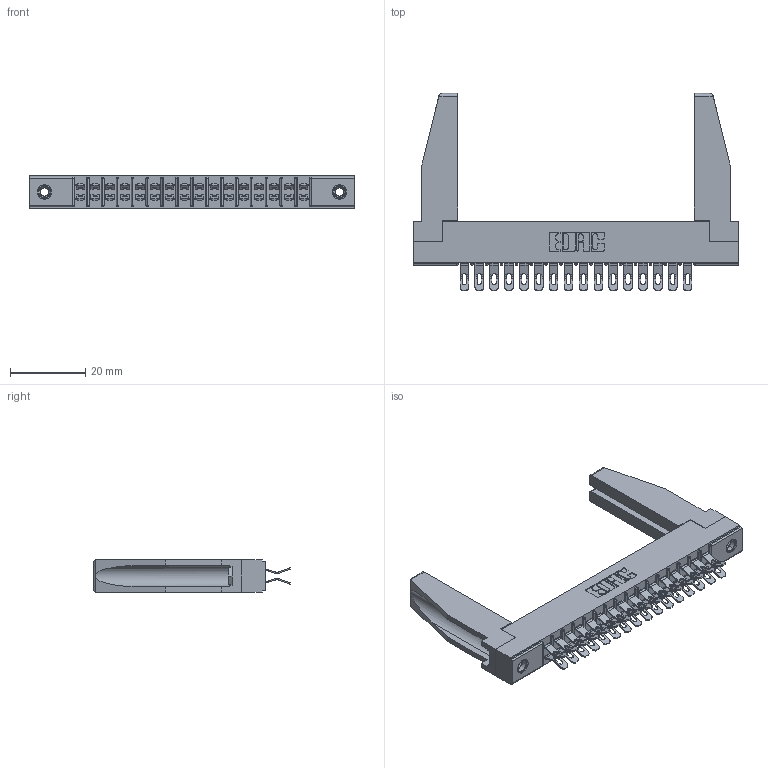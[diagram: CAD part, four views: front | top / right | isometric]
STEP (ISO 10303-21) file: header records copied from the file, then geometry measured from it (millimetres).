
FILE_DESCRIPTION (( 'STEP AP203' ), '1' );
FILE_NAME ('315-032-555-278.STEP', '2019-09-10T15:44:12', ( '' ), ( '' ), 'SwSTEP 2.0', 'SolidWorks 2016', '' );
FILE_SCHEMA (( 'CONFIG_CONTROL_DESIGN' ));
Length unit declared in the file: inch
Products named in the file (5): 305-290-001_555; 345-250-001_345-250-001-102; 315-032-555-278; 305 Part_.156 Dia; 307-220-078
Assembly tree (37 placements, depth 2):
  315-032-555-278
    305 Part_.156 Dia
    305-290-001_555  x32
    345-250-001_345-250-001-102  x2
    307-220-078  x2
Bounding box: 86.41 x 52.45 x 8.71 mm (x, y, z)
Volume: 9520.4 mm3; surface area: 14440.1 mm2
Topology: 37 solids, 37 shells, 2358 faces, 6966 edges, 4548 vertices
Faces by surface type: plane 1176, cylinder 1102, sphere 64, cone 12, torus 4
Entity records: 23552 total; most frequent: CARTESIAN_POINT 3922, ORIENTED_EDGE 3838, DIRECTION 3767, EDGE_CURVE 1919, LINE 1501, VECTOR 1501, VERTEX_POINT 1230, AXIS2_PLACEMENT_3D 1133
